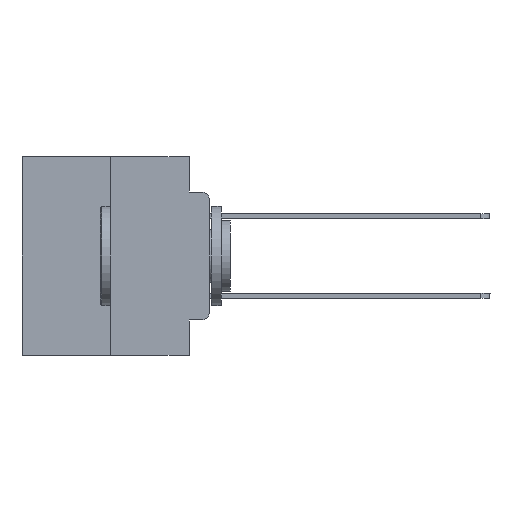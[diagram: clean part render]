
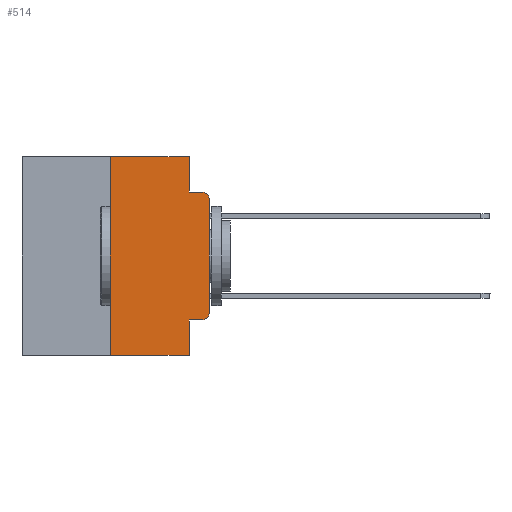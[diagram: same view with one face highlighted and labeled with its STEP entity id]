
A CAD part, left-side view. The second image highlights one B-rep face of the part: STEP entity #514.
In plain terms, the highlighted planar face has unit normal (-1, 0, 0).
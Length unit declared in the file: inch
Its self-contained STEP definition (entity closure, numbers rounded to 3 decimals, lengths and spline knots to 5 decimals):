
#86 = DIRECTION ( 'NONE',  ( 0., 0., 1. ) ) ;
#357 = LINE ( 'NONE', #17641, #20675 ) ;
#514 = ADVANCED_FACE ( 'NONE', ( #15144 ), #6780, .F. ) ;
#913 = CARTESIAN_POINT ( 'NONE',  ( 0., 0.051, -0.0885 ) ) ;
#1187 = CARTESIAN_POINT ( 'NONE',  ( 0., 0.02, -0.3915 ) ) ;
#1624 = CARTESIAN_POINT ( 'NONE',  ( 0., 0.051, 0. ) ) ;
#1697 = CARTESIAN_POINT ( 'NONE',  ( 0., 0.25, 0. ) ) ;
#1788 = ORIENTED_EDGE ( 'NONE', *, *, #26461, .F. ) ;
#2152 = CARTESIAN_POINT ( 'NONE',  ( 0., 0., -0.1085 ) ) ;
#2160 = DIRECTION ( 'NONE',  ( 0., 0., -1. ) ) ;
#2406 = LINE ( 'NONE', #17391, #24542 ) ;
#3264 = VERTEX_POINT ( 'NONE', #13042 ) ;
#3369 = AXIS2_PLACEMENT_3D ( 'NONE', #13173, #26525, #25969 ) ;
#3973 = CARTESIAN_POINT ( 'NONE',  ( 0., 0.02, -0.4115 ) ) ;
#4369 = VERTEX_POINT ( 'NONE', #3973 ) ;
#4690 = DIRECTION ( 'NONE',  ( 0., 0., -1. ) ) ;
#4710 = CARTESIAN_POINT ( 'NONE',  ( 0., 0.25, 0. ) ) ;
#5379 = VERTEX_POINT ( 'NONE', #10799 ) ;
#5427 = ORIENTED_EDGE ( 'NONE', *, *, #6984, .T. ) ;
#5959 = DIRECTION ( 'NONE',  ( 0., 0., -1. ) ) ;
#6780 = PLANE ( 'NONE',  #19644 ) ;
#6984 = EDGE_CURVE ( 'NONE', #3264, #17135, #2406, .T. ) ;
#7003 = ORIENTED_EDGE ( 'NONE', *, *, #18611, .T. ) ;
#7610 = EDGE_LOOP ( 'NONE', ( #5427, #18238, #25366, #1788, #10092, #16731, #7003, #15254, #14771, #16675 ) ) ;
#8383 = LINE ( 'NONE', #10960, #23030 ) ;
#8976 = DIRECTION ( 'NONE',  ( 0., -1., 0. ) ) ;
#9107 = EDGE_CURVE ( 'NONE', #17135, #20211, #11656, .T. ) ;
#9350 = EDGE_CURVE ( 'NONE', #4369, #3264, #18095, .T. ) ;
#9466 = CARTESIAN_POINT ( 'NONE',  ( 0., 0.02, -0.0885 ) ) ;
#9933 = DIRECTION ( 'NONE',  ( 0., -1., 0. ) ) ;
#10092 = ORIENTED_EDGE ( 'NONE', *, *, #18156, .F. ) ;
#10799 = CARTESIAN_POINT ( 'NONE',  ( 0., 0.25, -0.5 ) ) ;
#10960 = CARTESIAN_POINT ( 'NONE',  ( 0., 0.473, -0.5 ) ) ;
#11205 = DIRECTION ( 'NONE',  ( 0., 0., 1. ) ) ;
#11275 = CARTESIAN_POINT ( 'NONE',  ( 0., 0.051, -0.5 ) ) ;
#11656 = CIRCLE ( 'NONE', #3369, 0.02 ) ;
#12607 = LINE ( 'NONE', #1624, #13867 ) ;
#13042 = CARTESIAN_POINT ( 'NONE',  ( 0., 0., -0.3915 ) ) ;
#13173 = CARTESIAN_POINT ( 'NONE',  ( 0., 0.02, -0.1085 ) ) ;
#13753 = CARTESIAN_POINT ( 'NONE',  ( 0., 0.051, -0.0885 ) ) ;
#13867 = VECTOR ( 'NONE', #14457, 39.37008 ) ;
#14327 = VERTEX_POINT ( 'NONE', #13753 ) ;
#14457 = DIRECTION ( 'NONE',  ( 0., 0., -1. ) ) ;
#14771 = ORIENTED_EDGE ( 'NONE', *, *, #17477, .T. ) ;
#15144 = FACE_OUTER_BOUND ( 'NONE', #7610, .T. ) ;
#15254 = ORIENTED_EDGE ( 'NONE', *, *, #21842, .F. ) ;
#15570 = VERTEX_POINT ( 'NONE', #11275 ) ;
#16034 = LINE ( 'NONE', #913, #16992 ) ;
#16675 = ORIENTED_EDGE ( 'NONE', *, *, #9350, .T. ) ;
#16731 = ORIENTED_EDGE ( 'NONE', *, *, #24489, .F. ) ;
#16992 = VECTOR ( 'NONE', #25103, 39.37008 ) ;
#17019 = VERTEX_POINT ( 'NONE', #22927 ) ;
#17135 = VERTEX_POINT ( 'NONE', #2152 ) ;
#17162 = DIRECTION ( 'NONE',  ( 0., -1., 0. ) ) ;
#17391 = CARTESIAN_POINT ( 'NONE',  ( 0., 0., 0. ) ) ;
#17477 = EDGE_CURVE ( 'NONE', #17019, #4369, #21046, .T. ) ;
#17641 = CARTESIAN_POINT ( 'NONE',  ( 0., 0.051, 0. ) ) ;
#18095 = CIRCLE ( 'NONE', #20881, 0.02 ) ;
#18156 = EDGE_CURVE ( 'NONE', #27695, #26837, #19932, .T. ) ;
#18238 = ORIENTED_EDGE ( 'NONE', *, *, #9107, .T. ) ;
#18611 = EDGE_CURVE ( 'NONE', #5379, #15570, #8383, .T. ) ;
#18612 = CARTESIAN_POINT ( 'NONE',  ( 0., 0.051, 0. ) ) ;
#19644 = AXIS2_PLACEMENT_3D ( 'NONE', #23906, #22194, #2160 ) ;
#19932 = LINE ( 'NONE', #21945, #20200 ) ;
#20200 = VECTOR ( 'NONE', #8976, 39.37008 ) ;
#20211 = VERTEX_POINT ( 'NONE', #9466 ) ;
#20675 = VECTOR ( 'NONE', #4690, 39.37008 ) ;
#20881 = AXIS2_PLACEMENT_3D ( 'NONE', #1187, #25668, #5959 ) ;
#21046 = LINE ( 'NONE', #21325, #27102 ) ;
#21325 = CARTESIAN_POINT ( 'NONE',  ( 0., 0.051, -0.4115 ) ) ;
#21842 = EDGE_CURVE ( 'NONE', #17019, #15570, #357, .T. ) ;
#21945 = CARTESIAN_POINT ( 'NONE',  ( 0., 0.473, 0. ) ) ;
#22194 = DIRECTION ( 'NONE',  ( 1., 0., 0. ) ) ;
#22927 = CARTESIAN_POINT ( 'NONE',  ( 0., 0.051, -0.4115 ) ) ;
#23030 = VECTOR ( 'NONE', #17162, 39.37008 ) ;
#23727 = EDGE_CURVE ( 'NONE', #14327, #20211, #16034, .T. ) ;
#23888 = VECTOR ( 'NONE', #86, 39.37008 ) ;
#23906 = CARTESIAN_POINT ( 'NONE',  ( 0., 0.473, 0. ) ) ;
#24423 = LINE ( 'NONE', #4710, #23888 ) ;
#24489 = EDGE_CURVE ( 'NONE', #5379, #27695, #24423, .T. ) ;
#24542 = VECTOR ( 'NONE', #11205, 39.37008 ) ;
#25103 = DIRECTION ( 'NONE',  ( 0., -1., 0. ) ) ;
#25366 = ORIENTED_EDGE ( 'NONE', *, *, #23727, .F. ) ;
#25668 = DIRECTION ( 'NONE',  ( -1., 0., 0. ) ) ;
#25969 = DIRECTION ( 'NONE',  ( 0., 0., -1. ) ) ;
#26461 = EDGE_CURVE ( 'NONE', #26837, #14327, #12607, .T. ) ;
#26525 = DIRECTION ( 'NONE',  ( -1., 0., 0. ) ) ;
#26837 = VERTEX_POINT ( 'NONE', #18612 ) ;
#27102 = VECTOR ( 'NONE', #9933, 39.37008 ) ;
#27695 = VERTEX_POINT ( 'NONE', #1697 ) ;
